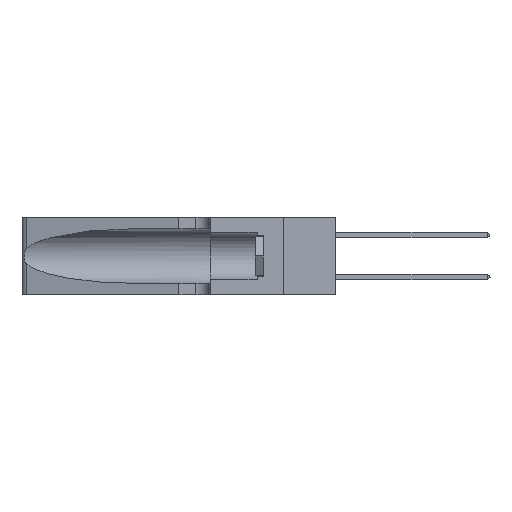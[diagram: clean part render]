
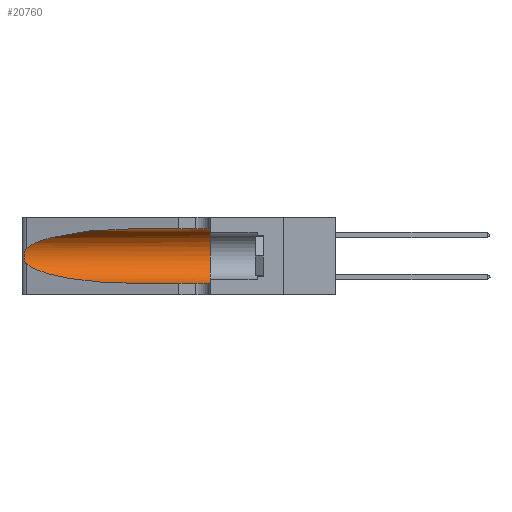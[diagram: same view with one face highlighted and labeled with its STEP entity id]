
A CAD part, left-side view. The second image highlights one B-rep face of the part: STEP entity #20760.
In plain terms, the highlighted cylindrical face has radius 3.308 mm (diameter 6.617 mm), a partial arc.
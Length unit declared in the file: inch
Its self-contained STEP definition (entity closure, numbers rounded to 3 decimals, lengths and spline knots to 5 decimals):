
#151 = CIRCLE ( 'NONE', #19800, 0.13025 ) ;
#380 = CARTESIAN_POINT ( 'NONE',  ( 0.1305, 0.72297, 0.31525 ) ) ;
#727 = VECTOR ( 'NONE', #17553, 39.37008 ) ;
#757 = B_SPLINE_CURVE_WITH_KNOTS ( 'NONE', 3,
 ( #33729, #30352, #4279, #24019, #36943, #4564, #40313, #33863, #37089, #26796, #26953, #14010, #30207, #20936 ),
 .UNSPECIFIED., .F., .F.,
 ( 4, 2, 2, 2, 2, 2, 4 ),
 ( 0., 0.00027, 0.00053, 0.00107, 0.0016, 0.00187, 0.00214 ),
 .UNSPECIFIED. ) ;
#1425 = EDGE_CURVE ( 'NONE', #26181, #40070, #8811, .T. ) ;
#1558 =( BOUNDED_CURVE ( )  B_SPLINE_CURVE ( 3, ( #380, #25629, #22922, #6308 ),
 .UNSPECIFIED., .F., .F. ) 
 B_SPLINE_CURVE_WITH_KNOTS ( ( 4, 4 ),
 ( 1.5708, 2.84003 ),
 .UNSPECIFIED. ) 
 CURVE ( )  GEOMETRIC_REPRESENTATION_ITEM ( )  RATIONAL_B_SPLINE_CURVE ( ( 1., 0.87, 0.87, 1. ) ) 
 REPRESENTATION_ITEM ( '' )  );
#1859 = CARTESIAN_POINT ( 'NONE',  ( 0.18966, 0.96281, 0.05475 ) ) ;
#3693 = ORIENTED_EDGE ( 'NONE', *, *, #37490, .T. ) ;
#3958 = DIRECTION ( 'NONE',  ( 0., -1., 0. ) ) ;
#4279 = CARTESIAN_POINT ( 'NONE',  ( 0.25639, 1.23184, 0.21858 ) ) ;
#4564 = CARTESIAN_POINT ( 'NONE',  ( 0.26018, 1.23835, 0.19895 ) ) ;
#6308 = CARTESIAN_POINT ( 'NONE',  ( 0.25487, 1.22718, 0.22369 ) ) ;
#7360 = VERTEX_POINT ( 'NONE', #37657 ) ;
#7585 = VERTEX_POINT ( 'NONE', #28969 ) ;
#8555 = ORIENTED_EDGE ( 'NONE', *, *, #19667, .T. ) ;
#8710 = ORIENTED_EDGE ( 'NONE', *, *, #1425, .T. ) ;
#8811 = LINE ( 'NONE', #10878, #727 ) ;
#9436 = DIRECTION ( 'NONE',  ( 0., 1., 0. ) ) ;
#10264 =( BOUNDED_CURVE ( )  B_SPLINE_CURVE ( 3, ( #40843, #11541, #1859, #33962 ),
 .UNSPECIFIED., .F., .T. ) 
 B_SPLINE_CURVE_WITH_KNOTS ( ( 4, 4 ),
 ( 3.44316, 4.71239 ),
 .UNSPECIFIED. ) 
 CURVE ( )  GEOMETRIC_REPRESENTATION_ITEM ( )  RATIONAL_B_SPLINE_CURVE ( ( 1., 0.87, 0.87, 1. ) ) 
 REPRESENTATION_ITEM ( '' )  );
#10878 = CARTESIAN_POINT ( 'NONE',  ( 0.1305, 1.61858, 0.05475 ) ) ;
#11541 = CARTESIAN_POINT ( 'NONE',  ( 0.2373, 1.15595, 0.08982 ) ) ;
#14010 = CARTESIAN_POINT ( 'NONE',  ( 0.25639, 1.23186, 0.15144 ) ) ;
#15413 = DIRECTION ( 'NONE',  ( 0., 0., 1. ) ) ;
#15962 = CARTESIAN_POINT ( 'NONE',  ( 0.1305, 0.35, 0.185 ) ) ;
#16276 = CARTESIAN_POINT ( 'NONE',  ( 0.1305, 0.35, 0.31525 ) ) ;
#17553 = DIRECTION ( 'NONE',  ( 0., -1., 0. ) ) ;
#17687 = CARTESIAN_POINT ( 'NONE',  ( 0.1305, 0.35, 0.05475 ) ) ;
#18958 = VERTEX_POINT ( 'NONE', #23750 ) ;
#19638 = ORIENTED_EDGE ( 'NONE', *, *, #37791, .T. ) ;
#19667 = EDGE_CURVE ( 'NONE', #7585, #18958, #757, .T. ) ;
#19715 = CARTESIAN_POINT ( 'NONE',  ( 0.1305, 0.72297, 0.05475 ) ) ;
#19800 = AXIS2_PLACEMENT_3D ( 'NONE', #15962, #9436, #15413 ) ;
#20239 = EDGE_CURVE ( 'NONE', #7360, #30667, #39444, .T. ) ;
#20320 = DIRECTION ( 'NONE',  ( 0., 0., -1. ) ) ;
#20760 = ADVANCED_FACE ( 'NONE', ( #27846 ), #29331, .F. ) ;
#20936 = CARTESIAN_POINT ( 'NONE',  ( 0.25487, 1.22718, 0.14631 ) ) ;
#21363 = VECTOR ( 'NONE', #3958, 39.37008 ) ;
#22922 = CARTESIAN_POINT ( 'NONE',  ( 0.2373, 1.15595, 0.28018 ) ) ;
#23134 = ORIENTED_EDGE ( 'NONE', *, *, #20239, .F. ) ;
#23750 = CARTESIAN_POINT ( 'NONE',  ( 0.25487, 1.22718, 0.14631 ) ) ;
#24019 = CARTESIAN_POINT ( 'NONE',  ( 0.25787, 1.23484, 0.2124 ) ) ;
#25130 = EDGE_LOOP ( 'NONE', ( #19638, #8555, #3693, #8710, #28500, #23134 ) ) ;
#25629 = CARTESIAN_POINT ( 'NONE',  ( 0.18966, 0.96281, 0.31525 ) ) ;
#25805 = DIRECTION ( 'NONE',  ( 0., -1., 0. ) ) ;
#26181 = VERTEX_POINT ( 'NONE', #19715 ) ;
#26347 = CARTESIAN_POINT ( 'NONE',  ( 0.1305, 1.61858, 0.31525 ) ) ;
#26796 = CARTESIAN_POINT ( 'NONE',  ( 0.25856, 1.23593, 0.16098 ) ) ;
#26953 = CARTESIAN_POINT ( 'NONE',  ( 0.25789, 1.23486, 0.15765 ) ) ;
#27846 = FACE_OUTER_BOUND ( 'NONE', #25130, .T. ) ;
#28500 = ORIENTED_EDGE ( 'NONE', *, *, #36316, .F. ) ;
#28969 = CARTESIAN_POINT ( 'NONE',  ( 0.25487, 1.22718, 0.22369 ) ) ;
#29331 = CYLINDRICAL_SURFACE ( 'NONE', #29677, 0.13025 ) ;
#29677 = AXIS2_PLACEMENT_3D ( 'NONE', #32150, #25805, #20320 ) ;
#30207 = CARTESIAN_POINT ( 'NONE',  ( 0.25555, 1.22993, 0.14849 ) ) ;
#30352 = CARTESIAN_POINT ( 'NONE',  ( 0.25555, 1.22994, 0.2215 ) ) ;
#30667 = VERTEX_POINT ( 'NONE', #16276 ) ;
#32150 = CARTESIAN_POINT ( 'NONE',  ( 0.1305, 1.61858, 0.185 ) ) ;
#33729 = CARTESIAN_POINT ( 'NONE',  ( 0.25487, 1.22718, 0.22369 ) ) ;
#33863 = CARTESIAN_POINT ( 'NONE',  ( 0.26075, 1.23896, 0.178 ) ) ;
#33962 = CARTESIAN_POINT ( 'NONE',  ( 0.1305, 0.72297, 0.05475 ) ) ;
#36316 = EDGE_CURVE ( 'NONE', #30667, #40070, #151, .T. ) ;
#36943 = CARTESIAN_POINT ( 'NONE',  ( 0.25854, 1.2359, 0.20912 ) ) ;
#37089 = CARTESIAN_POINT ( 'NONE',  ( 0.26017, 1.23833, 0.17102 ) ) ;
#37490 = EDGE_CURVE ( 'NONE', #18958, #26181, #10264, .T. ) ;
#37657 = CARTESIAN_POINT ( 'NONE',  ( 0.1305, 0.72297, 0.31525 ) ) ;
#37791 = EDGE_CURVE ( 'NONE', #7360, #7585, #1558, .T. ) ;
#39444 = LINE ( 'NONE', #26347, #21363 ) ;
#40070 = VERTEX_POINT ( 'NONE', #17687 ) ;
#40313 = CARTESIAN_POINT ( 'NONE',  ( 0.26075, 1.23896, 0.19203 ) ) ;
#40843 = CARTESIAN_POINT ( 'NONE',  ( 0.25487, 1.22718, 0.14631 ) ) ;
